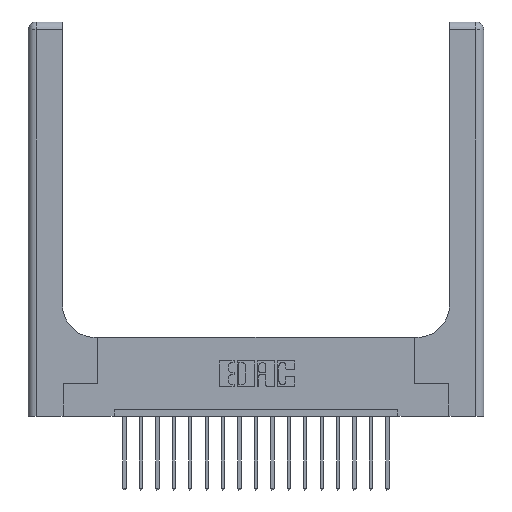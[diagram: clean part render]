
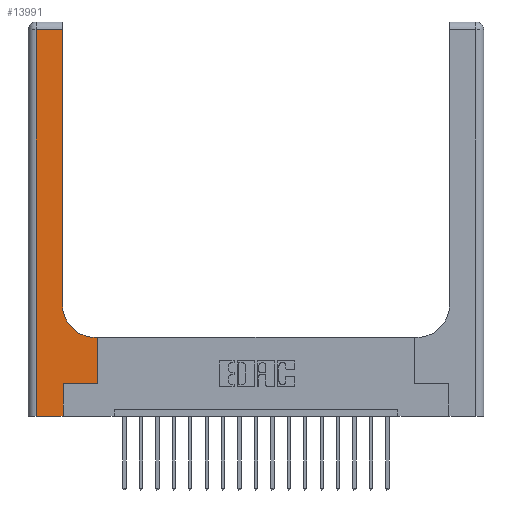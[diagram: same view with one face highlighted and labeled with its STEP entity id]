
A CAD part, top view. The second image highlights one B-rep face of the part: STEP entity #13991.
In plain terms, the highlighted planar face has unit normal (0, 0, 1).
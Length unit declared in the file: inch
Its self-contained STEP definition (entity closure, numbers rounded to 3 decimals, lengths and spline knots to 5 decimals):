
#37 = VECTOR ( 'NONE', #18095, 39.37008 ) ;
#293 = VERTEX_POINT ( 'NONE', #11454 ) ;
#311 = VERTEX_POINT ( 'NONE', #17383 ) ;
#363 = CARTESIAN_POINT ( 'NONE',  ( 0., 3., 0.37 ) ) ;
#423 = EDGE_CURVE ( 'NONE', #6143, #17839, #7576, .T. ) ;
#765 = LINE ( 'NONE', #8666, #16343 ) ;
#1062 = DIRECTION ( 'NONE',  ( 1., 0., 0. ) ) ;
#1316 = CARTESIAN_POINT ( 'NONE',  ( 0.06, 3., 0.37 ) ) ;
#1690 = EDGE_CURVE ( 'NONE', #311, #6143, #18563, .T. ) ;
#1839 = DIRECTION ( 'NONE',  ( -1., 0., 0. ) ) ;
#2269 = AXIS2_PLACEMENT_3D ( 'NONE', #363, #12241, #1839 ) ;
#2656 = DIRECTION ( 'NONE',  ( 0., 1., 0. ) ) ;
#3804 = ORIENTED_EDGE ( 'NONE', *, *, #6551, .T. ) ;
#4143 = VERTEX_POINT ( 'NONE', #9835 ) ;
#4516 = DIRECTION ( 'NONE',  ( -1., 0., 0. ) ) ;
#4715 = CARTESIAN_POINT ( 'NONE',  ( 0., 2.94, 0.37 ) ) ;
#4817 = CARTESIAN_POINT ( 'NONE',  ( 0.528, 0.6, 0.37 ) ) ;
#5002 = VECTOR ( 'NONE', #2656, 39.37008 ) ;
#5296 = DIRECTION ( 'NONE',  ( 0., 0., -1. ) ) ;
#5437 = ORIENTED_EDGE ( 'NONE', *, *, #16255, .T. ) ;
#5758 = EDGE_CURVE ( 'NONE', #14024, #293, #11101, .T. ) ;
#5826 = VERTEX_POINT ( 'NONE', #7227 ) ;
#5924 = CARTESIAN_POINT ( 'NONE',  ( 0.265, 0.25, 0.37 ) ) ;
#6006 = LINE ( 'NONE', #15029, #5002 ) ;
#6143 = VERTEX_POINT ( 'NONE', #13244 ) ;
#6193 = PLANE ( 'NONE',  #2269 ) ;
#6235 = EDGE_LOOP ( 'NONE', ( #7274, #11036, #9115, #3804, #14139, #17168, #7721, #7202, #5437 ) ) ;
#6511 = VECTOR ( 'NONE', #8325, 39.37008 ) ;
#6551 = EDGE_CURVE ( 'NONE', #4143, #12672, #765, .T. ) ;
#6723 = VECTOR ( 'NONE', #9464, 39.37008 ) ;
#6772 = CARTESIAN_POINT ( 'NONE',  ( 0.51, 0.85, 0.37 ) ) ;
#7202 = ORIENTED_EDGE ( 'NONE', *, *, #5758, .T. ) ;
#7227 = CARTESIAN_POINT ( 'NONE',  ( 0.265, 0.25, 0.37 ) ) ;
#7240 = VECTOR ( 'NONE', #7343, 39.37008 ) ;
#7274 = ORIENTED_EDGE ( 'NONE', *, *, #1690, .T. ) ;
#7343 = DIRECTION ( 'NONE',  ( 0., -1., 0. ) ) ;
#7576 = LINE ( 'NONE', #4715, #15314 ) ;
#7721 = ORIENTED_EDGE ( 'NONE', *, *, #14903, .T. ) ;
#8131 = LINE ( 'NONE', #18917, #11426 ) ;
#8325 = DIRECTION ( 'NONE',  ( -1., 0., 0. ) ) ;
#8666 = CARTESIAN_POINT ( 'NONE',  ( 0., 0., 0.37 ) ) ;
#9115 = ORIENTED_EDGE ( 'NONE', *, *, #10807, .T. ) ;
#9361 = FACE_OUTER_BOUND ( 'NONE', #6235, .T. ) ;
#9464 = DIRECTION ( 'NONE',  ( 0., 1., 0. ) ) ;
#9835 = CARTESIAN_POINT ( 'NONE',  ( 0.06, 0., 0.37 ) ) ;
#10083 = CIRCLE ( 'NONE', #16717, 0.25 ) ;
#10446 = CARTESIAN_POINT ( 'NONE',  ( 0.265, 0., 0.37 ) ) ;
#10807 = EDGE_CURVE ( 'NONE', #17839, #4143, #14878, .T. ) ;
#10948 = CARTESIAN_POINT ( 'NONE',  ( 0.26, 3., 0.37 ) ) ;
#11036 = ORIENTED_EDGE ( 'NONE', *, *, #423, .T. ) ;
#11101 = LINE ( 'NONE', #17140, #6511 ) ;
#11103 = DIRECTION ( 'NONE',  ( 0., 1., 0. ) ) ;
#11327 = DIRECTION ( 'NONE',  ( 1., 0., 0. ) ) ;
#11426 = VECTOR ( 'NONE', #11103, 39.37008 ) ;
#11454 = CARTESIAN_POINT ( 'NONE',  ( 0.51, 0.6, 0.37 ) ) ;
#11949 = VERTEX_POINT ( 'NONE', #16221 ) ;
#12241 = DIRECTION ( 'NONE',  ( 0., 0., -1. ) ) ;
#12672 = VERTEX_POINT ( 'NONE', #10446 ) ;
#13244 = CARTESIAN_POINT ( 'NONE',  ( 0.26, 2.94, 0.37 ) ) ;
#13349 = EDGE_CURVE ( 'NONE', #12672, #5826, #8131, .T. ) ;
#13991 = ADVANCED_FACE ( 'NONE', ( #9361 ), #6193, .F. ) ;
#14024 = VERTEX_POINT ( 'NONE', #4817 ) ;
#14139 = ORIENTED_EDGE ( 'NONE', *, *, #13349, .T. ) ;
#14878 = LINE ( 'NONE', #1316, #7240 ) ;
#14903 = EDGE_CURVE ( 'NONE', #11949, #14024, #6006, .T. ) ;
#15029 = CARTESIAN_POINT ( 'NONE',  ( 0.528, 0.25, 0.37 ) ) ;
#15314 = VECTOR ( 'NONE', #4516, 39.37008 ) ;
#16221 = CARTESIAN_POINT ( 'NONE',  ( 0.528, 0.25, 0.37 ) ) ;
#16255 = EDGE_CURVE ( 'NONE', #293, #311, #10083, .T. ) ;
#16343 = VECTOR ( 'NONE', #1062, 39.37008 ) ;
#16415 = LINE ( 'NONE', #5924, #37 ) ;
#16717 = AXIS2_PLACEMENT_3D ( 'NONE', #6772, #5296, #11327 ) ;
#17140 = CARTESIAN_POINT ( 'NONE',  ( 0.26, 0.6, 0.37 ) ) ;
#17168 = ORIENTED_EDGE ( 'NONE', *, *, #18466, .T. ) ;
#17383 = CARTESIAN_POINT ( 'NONE',  ( 0.26, 0.85, 0.37 ) ) ;
#17839 = VERTEX_POINT ( 'NONE', #19060 ) ;
#18095 = DIRECTION ( 'NONE',  ( 1., 0., 0. ) ) ;
#18466 = EDGE_CURVE ( 'NONE', #5826, #11949, #16415, .T. ) ;
#18563 = LINE ( 'NONE', #10948, #6723 ) ;
#18917 = CARTESIAN_POINT ( 'NONE',  ( 0.265, 0., 0.37 ) ) ;
#19060 = CARTESIAN_POINT ( 'NONE',  ( 0.06, 2.94, 0.37 ) ) ;
